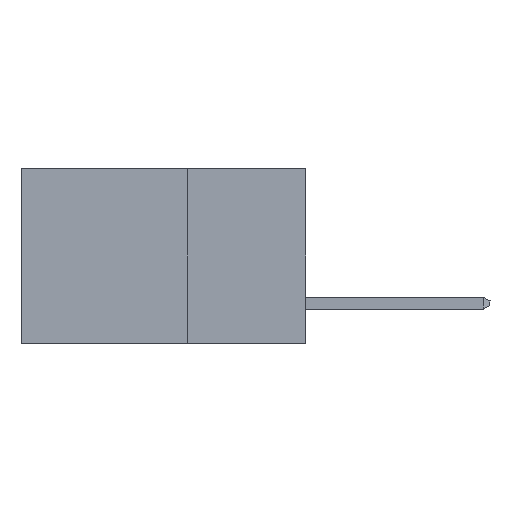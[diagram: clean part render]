
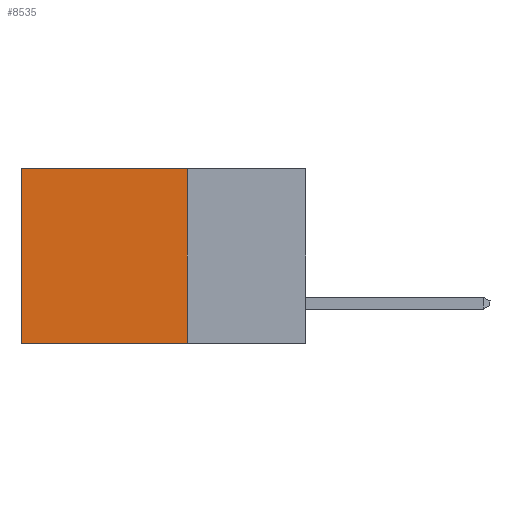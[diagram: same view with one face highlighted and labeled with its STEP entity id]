
A CAD part, left-side view. The second image highlights one B-rep face of the part: STEP entity #8535.
In plain terms, the highlighted planar face has unit normal (-1, 0, 0).
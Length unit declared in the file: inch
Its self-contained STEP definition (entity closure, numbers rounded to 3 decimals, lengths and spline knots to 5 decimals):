
#67 = VERTEX_POINT ( 'NONE', #9927 ) ;
#749 = VECTOR ( 'NONE', #7390, 39.37008 ) ;
#1398 = VERTEX_POINT ( 'NONE', #6631 ) ;
#2535 = DIRECTION ( 'NONE',  ( 0., 0., -1. ) ) ;
#2927 = ORIENTED_EDGE ( 'NONE', *, *, #12455, .T. ) ;
#3470 = LINE ( 'NONE', #12662, #749 ) ;
#3485 = VECTOR ( 'NONE', #6878, 39.37008 ) ;
#4655 = ORIENTED_EDGE ( 'NONE', *, *, #9633, .F. ) ;
#5657 = CARTESIAN_POINT ( 'NONE',  ( 0.298, 0.25, 0. ) ) ;
#5953 = ORIENTED_EDGE ( 'NONE', *, *, #9315, .F. ) ;
#6144 = FACE_OUTER_BOUND ( 'NONE', #10169, .T. ) ;
#6227 = LINE ( 'NONE', #10964, #3485 ) ;
#6376 = CARTESIAN_POINT ( 'NONE',  ( 0.298, 0.6, 0. ) ) ;
#6631 = CARTESIAN_POINT ( 'NONE',  ( 0.298, 0.6, -0.37 ) ) ;
#6676 = LINE ( 'NONE', #12044, #10230 ) ;
#6698 = DIRECTION ( 'NONE',  ( 1., 0., 0. ) ) ;
#6874 = DIRECTION ( 'NONE',  ( 0., 1., 0. ) ) ;
#6878 = DIRECTION ( 'NONE',  ( 0., 1., 0. ) ) ;
#7149 = CARTESIAN_POINT ( 'NONE',  ( 0.298, 0.6, 0. ) ) ;
#7390 = DIRECTION ( 'NONE',  ( 0., 0., -1. ) ) ;
#8535 = ADVANCED_FACE ( 'NONE', ( #6144 ), #8715, .F. ) ;
#8715 = PLANE ( 'NONE',  #11221 ) ;
#8897 = LINE ( 'NONE', #6376, #9691 ) ;
#9315 = EDGE_CURVE ( 'NONE', #67, #1398, #6227, .T. ) ;
#9633 = EDGE_CURVE ( 'NONE', #12767, #67, #3470, .T. ) ;
#9691 = VECTOR ( 'NONE', #11584, 39.37008 ) ;
#9927 = CARTESIAN_POINT ( 'NONE',  ( 0.298, 0.25, -0.37 ) ) ;
#10169 = EDGE_LOOP ( 'NONE', ( #2927, #5953, #4655, #11096 ) ) ;
#10230 = VECTOR ( 'NONE', #6874, 39.37008 ) ;
#10964 = CARTESIAN_POINT ( 'NONE',  ( 0.298, 0.25, -0.37 ) ) ;
#11096 = ORIENTED_EDGE ( 'NONE', *, *, #11227, .T. ) ;
#11221 = AXIS2_PLACEMENT_3D ( 'NONE', #5657, #6698, #2535 ) ;
#11227 = EDGE_CURVE ( 'NONE', #12767, #13267, #6676, .T. ) ;
#11584 = DIRECTION ( 'NONE',  ( 0., 0., -1. ) ) ;
#12044 = CARTESIAN_POINT ( 'NONE',  ( 0.298, 0.25, 0. ) ) ;
#12455 = EDGE_CURVE ( 'NONE', #13267, #1398, #8897, .T. ) ;
#12662 = CARTESIAN_POINT ( 'NONE',  ( 0.298, 0.25, 0. ) ) ;
#12767 = VERTEX_POINT ( 'NONE', #12995 ) ;
#12995 = CARTESIAN_POINT ( 'NONE',  ( 0.298, 0.25, 0. ) ) ;
#13267 = VERTEX_POINT ( 'NONE', #7149 ) ;
